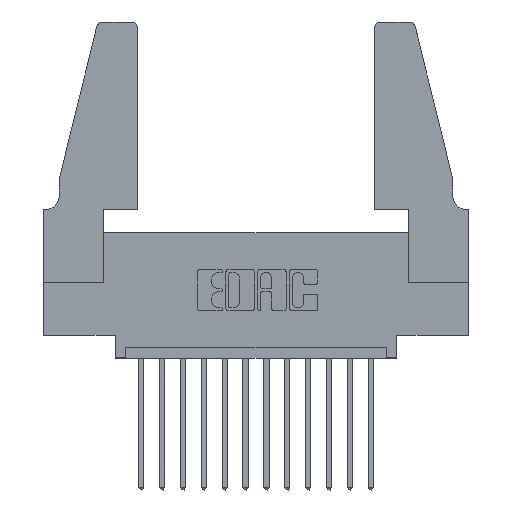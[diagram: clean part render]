
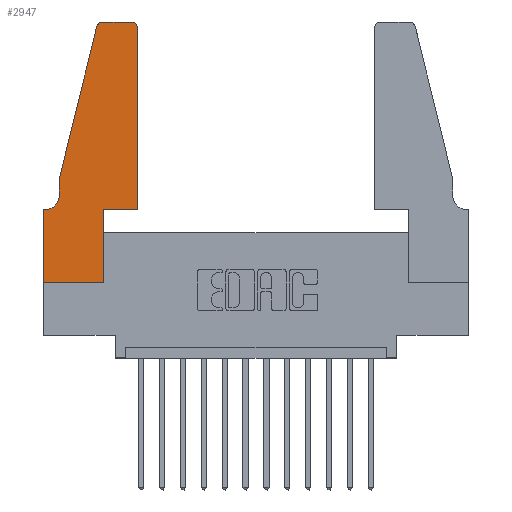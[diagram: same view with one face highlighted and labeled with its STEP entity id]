
A CAD part, top view. The second image highlights one B-rep face of the part: STEP entity #2947.
In plain terms, the highlighted planar face has unit normal (0, 0, 1).
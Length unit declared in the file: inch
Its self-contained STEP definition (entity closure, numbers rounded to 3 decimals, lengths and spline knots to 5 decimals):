
#5 = VERTEX_POINT ( 'NONE', #2541 ) ;
#8 = LINE ( 'NONE', #9540, #15050 ) ;
#339 = CARTESIAN_POINT ( 'NONE',  ( 0.0755, 0.5, 0.37 ) ) ;
#351 = EDGE_CURVE ( 'NONE', #1560, #4568, #13118, .T. ) ;
#539 = LINE ( 'NONE', #3483, #2941 ) ;
#550 = EDGE_CURVE ( 'NONE', #3967, #5, #5626, .T. ) ;
#719 = AXIS2_PLACEMENT_3D ( 'NONE', #6019, #10603, #8314 ) ;
#746 = DIRECTION ( 'NONE',  ( 0., 0., 1. ) ) ;
#910 = VERTEX_POINT ( 'NONE', #14790 ) ;
#1018 = DIRECTION ( 'NONE',  ( 1., 0., 0. ) ) ;
#1183 = AXIS2_PLACEMENT_3D ( 'NONE', #12558, #746, #15212 ) ;
#1230 = ORIENTED_EDGE ( 'NONE', *, *, #7748, .T. ) ;
#1515 = ORIENTED_EDGE ( 'NONE', *, *, #4281, .T. ) ;
#1549 = DIRECTION ( 'NONE',  ( -1., 0., 0. ) ) ;
#1560 = VERTEX_POINT ( 'NONE', #4967 ) ;
#1784 = EDGE_CURVE ( 'NONE', #6591, #910, #9730, .T. ) ;
#1887 = VECTOR ( 'NONE', #4473, 39.37008 ) ;
#2201 = CARTESIAN_POINT ( 'NONE',  ( 0.2865, 0., 0.37 ) ) ;
#2212 = DIRECTION ( 'NONE',  ( 0., 0., 1. ) ) ;
#2353 = VECTOR ( 'NONE', #6999, 39.37008 ) ;
#2541 = CARTESIAN_POINT ( 'NONE',  ( 0.0055, 0.35, 0.37 ) ) ;
#2552 = VECTOR ( 'NONE', #1549, 39.37008 ) ;
#2941 = VECTOR ( 'NONE', #1018, 39.37008 ) ;
#2947 = ADVANCED_FACE ( 'NONE', ( #13819 ), #13756, .T. ) ;
#3026 = AXIS2_PLACEMENT_3D ( 'NONE', #13040, #15006, #4534 ) ;
#3309 = ORIENTED_EDGE ( 'NONE', *, *, #11895, .T. ) ;
#3332 = VERTEX_POINT ( 'NONE', #13857 ) ;
#3460 = AXIS2_PLACEMENT_3D ( 'NONE', #11521, #2212, #11729 ) ;
#3483 = CARTESIAN_POINT ( 'NONE',  ( 0., 0., 0.37 ) ) ;
#3615 = ORIENTED_EDGE ( 'NONE', *, *, #550, .T. ) ;
#3752 = CARTESIAN_POINT ( 'NONE',  ( 0.4505, 0.35, 0.37 ) ) ;
#3967 = VERTEX_POINT ( 'NONE', #11488 ) ;
#4035 = ORIENTED_EDGE ( 'NONE', *, *, #14246, .T. ) ;
#4239 = CARTESIAN_POINT ( 'NONE',  ( 0., 0., 0.37 ) ) ;
#4281 = EDGE_CURVE ( 'NONE', #12393, #3967, #4815, .T. ) ;
#4473 = DIRECTION ( 'NONE',  ( -1., 0., 0. ) ) ;
#4530 = VECTOR ( 'NONE', #11216, 39.37008 ) ;
#4534 = DIRECTION ( 'NONE',  ( -1., 0., 0. ) ) ;
#4568 = VERTEX_POINT ( 'NONE', #4239 ) ;
#4569 = LINE ( 'NONE', #10891, #2552 ) ;
#4815 = LINE ( 'NONE', #339, #9847 ) ;
#4967 = CARTESIAN_POINT ( 'NONE',  ( 0., 0.35, 0.37 ) ) ;
#5626 = CIRCLE ( 'NONE', #3026, 0.07 ) ;
#5678 = VERTEX_POINT ( 'NONE', #2201 ) ;
#6019 = CARTESIAN_POINT ( 'NONE',  ( 0.4205, 1.22, 0.37 ) ) ;
#6275 = DIRECTION ( 'NONE',  ( 1., 0., 0. ) ) ;
#6323 = DIRECTION ( 'NONE',  ( 0., -1., 0. ) ) ;
#6555 = EDGE_CURVE ( 'NONE', #11387, #6591, #6606, .T. ) ;
#6591 = VERTEX_POINT ( 'NONE', #10148 ) ;
#6606 = LINE ( 'NONE', #3752, #11436 ) ;
#6872 = CARTESIAN_POINT ( 'NONE',  ( 0., 0., 0.37 ) ) ;
#6947 = EDGE_CURVE ( 'NONE', #5, #1560, #4569, .T. ) ;
#6999 = DIRECTION ( 'NONE',  ( 0., 1., 0. ) ) ;
#7551 = ORIENTED_EDGE ( 'NONE', *, *, #1784, .T. ) ;
#7597 = ORIENTED_EDGE ( 'NONE', *, *, #6947, .T. ) ;
#7748 = EDGE_CURVE ( 'NONE', #5678, #11387, #14248, .T. ) ;
#7773 = CIRCLE ( 'NONE', #3460, 0.03 ) ;
#8314 = DIRECTION ( 'NONE',  ( 1., 0., 0. ) ) ;
#8735 = CARTESIAN_POINT ( 'NONE',  ( 0.25487, 1.22718, 0.37 ) ) ;
#9013 = ORIENTED_EDGE ( 'NONE', *, *, #13681, .T. ) ;
#9388 = ORIENTED_EDGE ( 'NONE', *, *, #11425, .T. ) ;
#9404 = CIRCLE ( 'NONE', #719, 0.03 ) ;
#9540 = CARTESIAN_POINT ( 'NONE',  ( 0.0755, 0.5, 0.37 ) ) ;
#9693 = DIRECTION ( 'NONE',  ( -0.239, -0.971, 0. ) ) ;
#9730 = LINE ( 'NONE', #9903, #4530 ) ;
#9847 = VECTOR ( 'NONE', #6323, 39.37008 ) ;
#9903 = CARTESIAN_POINT ( 'NONE',  ( 0.4505, 0.35, 0.37 ) ) ;
#10148 = CARTESIAN_POINT ( 'NONE',  ( 0.4505, 0.35, 0.37 ) ) ;
#10394 = CARTESIAN_POINT ( 'NONE',  ( 0.2605, 1.25, 0.37 ) ) ;
#10603 = DIRECTION ( 'NONE',  ( 0., 0., 1. ) ) ;
#10891 = CARTESIAN_POINT ( 'NONE',  ( 0.0755, 0.35, 0.37 ) ) ;
#11216 = DIRECTION ( 'NONE',  ( 0., 1., 0. ) ) ;
#11387 = VERTEX_POINT ( 'NONE', #12235 ) ;
#11425 = EDGE_CURVE ( 'NONE', #3332, #13286, #13393, .T. ) ;
#11436 = VECTOR ( 'NONE', #6275, 39.37008 ) ;
#11488 = CARTESIAN_POINT ( 'NONE',  ( 0.0755, 0.42, 0.37 ) ) ;
#11521 = CARTESIAN_POINT ( 'NONE',  ( 0.284, 1.22, 0.37 ) ) ;
#11729 = DIRECTION ( 'NONE',  ( 1., 0., 0. ) ) ;
#11895 = EDGE_CURVE ( 'NONE', #12927, #12393, #8, .T. ) ;
#11897 = CARTESIAN_POINT ( 'NONE',  ( 0.284, 1.25, 0.37 ) ) ;
#12235 = CARTESIAN_POINT ( 'NONE',  ( 0.2865, 0.35, 0.37 ) ) ;
#12393 = VERTEX_POINT ( 'NONE', #14418 ) ;
#12429 = ORIENTED_EDGE ( 'NONE', *, *, #6555, .T. ) ;
#12558 = CARTESIAN_POINT ( 'NONE',  ( 0., 0.35, 0.37 ) ) ;
#12927 = VERTEX_POINT ( 'NONE', #8735 ) ;
#13040 = CARTESIAN_POINT ( 'NONE',  ( 0.0055, 0.42, 0.37 ) ) ;
#13118 = LINE ( 'NONE', #6872, #15165 ) ;
#13194 = EDGE_CURVE ( 'NONE', #13286, #12927, #7773, .T. ) ;
#13286 = VERTEX_POINT ( 'NONE', #11897 ) ;
#13393 = LINE ( 'NONE', #10394, #1887 ) ;
#13681 = EDGE_CURVE ( 'NONE', #4568, #5678, #539, .T. ) ;
#13756 = PLANE ( 'NONE',  #1183 ) ;
#13807 = ORIENTED_EDGE ( 'NONE', *, *, #351, .T. ) ;
#13819 = FACE_OUTER_BOUND ( 'NONE', #14937, .T. ) ;
#13857 = CARTESIAN_POINT ( 'NONE',  ( 0.4205, 1.25, 0.37 ) ) ;
#14246 = EDGE_CURVE ( 'NONE', #910, #3332, #9404, .T. ) ;
#14248 = LINE ( 'NONE', #14298, #2353 ) ;
#14298 = CARTESIAN_POINT ( 'NONE',  ( 0.2865, 0.35, 0.37 ) ) ;
#14418 = CARTESIAN_POINT ( 'NONE',  ( 0.0755, 0.5, 0.37 ) ) ;
#14790 = CARTESIAN_POINT ( 'NONE',  ( 0.4505, 1.22, 0.37 ) ) ;
#14908 = ORIENTED_EDGE ( 'NONE', *, *, #13194, .T. ) ;
#14937 = EDGE_LOOP ( 'NONE', ( #9388, #14908, #3309, #1515, #3615, #7597, #13807, #9013, #1230, #12429, #7551, #4035 ) ) ;
#15006 = DIRECTION ( 'NONE',  ( 0., 0., -1. ) ) ;
#15050 = VECTOR ( 'NONE', #9693, 39.37008 ) ;
#15165 = VECTOR ( 'NONE', #15225, 39.37008 ) ;
#15212 = DIRECTION ( 'NONE',  ( 1., 0., 0. ) ) ;
#15225 = DIRECTION ( 'NONE',  ( 0., -1., 0. ) ) ;
